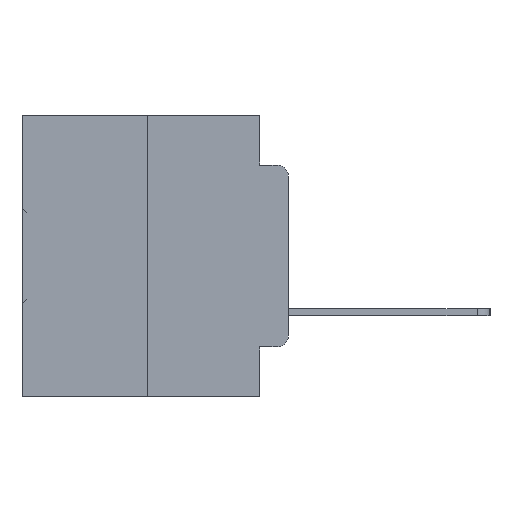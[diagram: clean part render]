
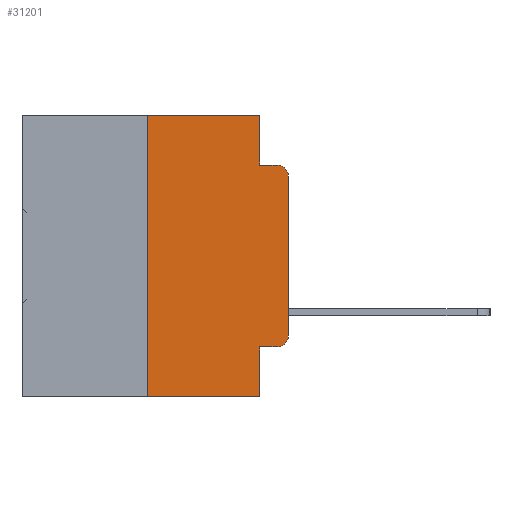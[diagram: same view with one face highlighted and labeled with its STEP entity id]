
A CAD part, left-side view. The second image highlights one B-rep face of the part: STEP entity #31201.
In plain terms, the highlighted planar face has unit normal (-1, 0, 0).
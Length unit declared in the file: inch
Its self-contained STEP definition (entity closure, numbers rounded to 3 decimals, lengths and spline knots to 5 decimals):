
#50 = EDGE_CURVE ( 'NONE', #27563, #7623, #29884, .T. ) ;
#520 = DIRECTION ( 'NONE',  ( 0., 0., -1. ) ) ;
#2881 = PLANE ( 'NONE',  #22641 ) ;
#3418 = ORIENTED_EDGE ( 'NONE', *, *, #8619, .F. ) ;
#3775 = CARTESIAN_POINT ( 'NONE',  ( 0., 0., -0.1085 ) ) ;
#3894 = DIRECTION ( 'NONE',  ( 0., 0., -1. ) ) ;
#4137 = CARTESIAN_POINT ( 'NONE',  ( 0., 0.051, -0.4115 ) ) ;
#4497 = CIRCLE ( 'NONE', #14899, 0.02 ) ;
#5310 = EDGE_CURVE ( 'NONE', #33193, #27553, #27128, .T. ) ;
#5992 = EDGE_CURVE ( 'NONE', #14374, #27553, #4497, .T. ) ;
#6288 = CARTESIAN_POINT ( 'NONE',  ( 0., 0.02, -0.4115 ) ) ;
#6297 = LINE ( 'NONE', #17160, #33387 ) ;
#6435 = EDGE_CURVE ( 'NONE', #11977, #7623, #18661, .T. ) ;
#6452 = DIRECTION ( 'NONE',  ( -1., 0., 0. ) ) ;
#6587 = DIRECTION ( 'NONE',  ( 0., 0., 1. ) ) ;
#7623 = VERTEX_POINT ( 'NONE', #28881 ) ;
#8069 = AXIS2_PLACEMENT_3D ( 'NONE', #14232, #32416, #16845 ) ;
#8185 = ORIENTED_EDGE ( 'NONE', *, *, #5310, .F. ) ;
#8191 = VECTOR ( 'NONE', #24937, 39.37008 ) ;
#8452 = DIRECTION ( 'NONE',  ( 0., 0., -1. ) ) ;
#8456 = VERTEX_POINT ( 'NONE', #6288 ) ;
#8619 = EDGE_CURVE ( 'NONE', #31597, #27551, #15318, .T. ) ;
#8676 = DIRECTION ( 'NONE',  ( 0., -1., 0. ) ) ;
#9594 = FACE_OUTER_BOUND ( 'NONE', #12663, .T. ) ;
#10750 = ORIENTED_EDGE ( 'NONE', *, *, #17132, .F. ) ;
#11116 = CARTESIAN_POINT ( 'NONE',  ( 0., 0., 0. ) ) ;
#11149 = ORIENTED_EDGE ( 'NONE', *, *, #15635, .T. ) ;
#11201 = CARTESIAN_POINT ( 'NONE',  ( 0., 0.051, 0. ) ) ;
#11402 = CARTESIAN_POINT ( 'NONE',  ( 0., 0.051, -0.0885 ) ) ;
#11787 = VECTOR ( 'NONE', #22716, 39.37008 ) ;
#11977 = VERTEX_POINT ( 'NONE', #27903 ) ;
#12650 = LINE ( 'NONE', #4137, #11787 ) ;
#12663 = EDGE_LOOP ( 'NONE', ( #11149, #19709, #8185, #22141, #3418, #10750, #19318, #33946, #22565, #31950 ) ) ;
#13547 = VECTOR ( 'NONE', #26708, 39.37008 ) ;
#13953 = CARTESIAN_POINT ( 'NONE',  ( 0., 0.25, -0.5 ) ) ;
#14232 = CARTESIAN_POINT ( 'NONE',  ( 0., 0.02, -0.3915 ) ) ;
#14374 = VERTEX_POINT ( 'NONE', #3775 ) ;
#14890 = CARTESIAN_POINT ( 'NONE',  ( 0., 0.473, -0.5 ) ) ;
#14899 = AXIS2_PLACEMENT_3D ( 'NONE', #22243, #6452, #24887 ) ;
#14955 = CARTESIAN_POINT ( 'NONE',  ( 0., 0.473, 0. ) ) ;
#15318 = LINE ( 'NONE', #14955, #28326 ) ;
#15635 = EDGE_CURVE ( 'NONE', #18532, #14374, #27346, .T. ) ;
#16845 = DIRECTION ( 'NONE',  ( 0., 0., -1. ) ) ;
#17132 = EDGE_CURVE ( 'NONE', #27563, #31597, #6297, .T. ) ;
#17160 = CARTESIAN_POINT ( 'NONE',  ( 0., 0.25, 0. ) ) ;
#17273 = CARTESIAN_POINT ( 'NONE',  ( 0., 0.051, 0. ) ) ;
#17581 = DIRECTION ( 'NONE',  ( 0., -1., 0. ) ) ;
#18532 = VERTEX_POINT ( 'NONE', #28611 ) ;
#18661 = LINE ( 'NONE', #19285, #31675 ) ;
#18881 = EDGE_CURVE ( 'NONE', #27551, #33193, #27995, .T. ) ;
#19285 = CARTESIAN_POINT ( 'NONE',  ( 0., 0.051, 0. ) ) ;
#19318 = ORIENTED_EDGE ( 'NONE', *, *, #50, .T. ) ;
#19709 = ORIENTED_EDGE ( 'NONE', *, *, #5992, .T. ) ;
#20730 = CARTESIAN_POINT ( 'NONE',  ( 0., 0.25, 0. ) ) ;
#21098 = VECTOR ( 'NONE', #3894, 39.37008 ) ;
#21526 = CARTESIAN_POINT ( 'NONE',  ( 0., 0.473, 0. ) ) ;
#22141 = ORIENTED_EDGE ( 'NONE', *, *, #18881, .F. ) ;
#22243 = CARTESIAN_POINT ( 'NONE',  ( 0., 0.02, -0.1085 ) ) ;
#22565 = ORIENTED_EDGE ( 'NONE', *, *, #29961, .T. ) ;
#22641 = AXIS2_PLACEMENT_3D ( 'NONE', #21526, #24148, #8452 ) ;
#22716 = DIRECTION ( 'NONE',  ( 0., -1., 0. ) ) ;
#24148 = DIRECTION ( 'NONE',  ( 1., 0., 0. ) ) ;
#24887 = DIRECTION ( 'NONE',  ( 0., 0., -1. ) ) ;
#24937 = DIRECTION ( 'NONE',  ( 0., -1., 0. ) ) ;
#26708 = DIRECTION ( 'NONE',  ( 0., 0., 1. ) ) ;
#27128 = LINE ( 'NONE', #11402, #33214 ) ;
#27346 = LINE ( 'NONE', #11116, #13547 ) ;
#27551 = VERTEX_POINT ( 'NONE', #11201 ) ;
#27553 = VERTEX_POINT ( 'NONE', #29503 ) ;
#27563 = VERTEX_POINT ( 'NONE', #13953 ) ;
#27903 = CARTESIAN_POINT ( 'NONE',  ( 0., 0.051, -0.4115 ) ) ;
#27995 = LINE ( 'NONE', #17273, #21098 ) ;
#28231 = EDGE_CURVE ( 'NONE', #8456, #18532, #30698, .T. ) ;
#28326 = VECTOR ( 'NONE', #17581, 39.37008 ) ;
#28611 = CARTESIAN_POINT ( 'NONE',  ( 0., 0., -0.3915 ) ) ;
#28881 = CARTESIAN_POINT ( 'NONE',  ( 0., 0.051, -0.5 ) ) ;
#29503 = CARTESIAN_POINT ( 'NONE',  ( 0., 0.02, -0.0885 ) ) ;
#29884 = LINE ( 'NONE', #14890, #8191 ) ;
#29961 = EDGE_CURVE ( 'NONE', #11977, #8456, #12650, .T. ) ;
#30698 = CIRCLE ( 'NONE', #8069, 0.02 ) ;
#31201 = ADVANCED_FACE ( 'NONE', ( #9594 ), #2881, .F. ) ;
#31597 = VERTEX_POINT ( 'NONE', #20730 ) ;
#31675 = VECTOR ( 'NONE', #520, 39.37008 ) ;
#31950 = ORIENTED_EDGE ( 'NONE', *, *, #28231, .T. ) ;
#32008 = CARTESIAN_POINT ( 'NONE',  ( 0., 0.051, -0.0885 ) ) ;
#32416 = DIRECTION ( 'NONE',  ( -1., 0., 0. ) ) ;
#33193 = VERTEX_POINT ( 'NONE', #32008 ) ;
#33214 = VECTOR ( 'NONE', #8676, 39.37008 ) ;
#33387 = VECTOR ( 'NONE', #6587, 39.37008 ) ;
#33946 = ORIENTED_EDGE ( 'NONE', *, *, #6435, .F. ) ;
